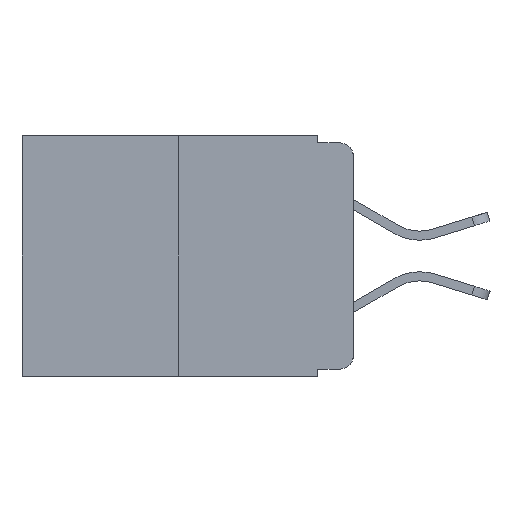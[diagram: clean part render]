
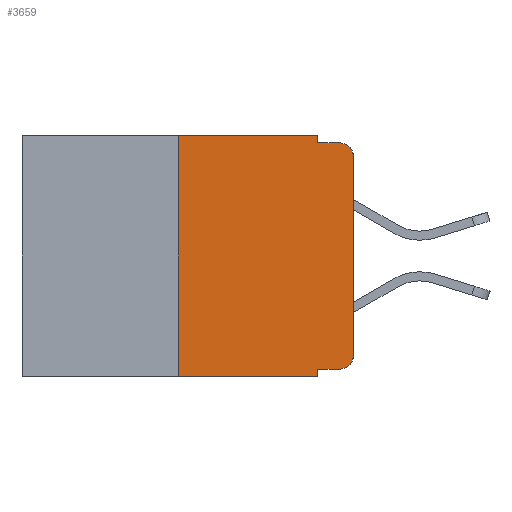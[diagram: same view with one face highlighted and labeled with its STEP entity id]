
A CAD part, left-side view. The second image highlights one B-rep face of the part: STEP entity #3659.
In plain terms, the highlighted planar face has unit normal (-1, 0, 0).
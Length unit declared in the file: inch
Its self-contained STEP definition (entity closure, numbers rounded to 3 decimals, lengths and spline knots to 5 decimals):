
#132 = VERTEX_POINT ( 'NONE', #7792 ) ;
#161 = CARTESIAN_POINT ( 'NONE',  ( 0., 0.473, 0. ) ) ;
#556 = CARTESIAN_POINT ( 'NONE',  ( 0., 0.02, -0.03 ) ) ;
#569 = FACE_OUTER_BOUND ( 'NONE', #10077, .T. ) ;
#776 = VECTOR ( 'NONE', #2933, 39.37008 ) ;
#932 = AXIS2_PLACEMENT_3D ( 'NONE', #6348, #8882, #5397 ) ;
#1039 = LINE ( 'NONE', #8646, #12114 ) ;
#1228 = VERTEX_POINT ( 'NONE', #4421 ) ;
#1411 = VERTEX_POINT ( 'NONE', #13259 ) ;
#1465 = VERTEX_POINT ( 'NONE', #2578 ) ;
#1787 = CIRCLE ( 'NONE', #10687, 0.02 ) ;
#1833 = CARTESIAN_POINT ( 'NONE',  ( 0., 0.25, -0.343 ) ) ;
#1888 = DIRECTION ( 'NONE',  ( -1., 0., 0. ) ) ;
#2293 = LINE ( 'NONE', #7137, #13174 ) ;
#2578 = CARTESIAN_POINT ( 'NONE',  ( 0., 0.051, -0.333 ) ) ;
#2852 = PLANE ( 'NONE',  #932 ) ;
#2933 = DIRECTION ( 'NONE',  ( 0., -1., 0. ) ) ;
#2960 = VERTEX_POINT ( 'NONE', #14194 ) ;
#3230 = DIRECTION ( 'NONE',  ( 0., -1., 0. ) ) ;
#3345 = DIRECTION ( 'NONE',  ( 0., -1., 0. ) ) ;
#3346 = ORIENTED_EDGE ( 'NONE', *, *, #15457, .T. ) ;
#3429 = VERTEX_POINT ( 'NONE', #15495 ) ;
#3498 = EDGE_CURVE ( 'NONE', #1465, #132, #1039, .T. ) ;
#3659 = ADVANCED_FACE ( 'NONE', ( #569 ), #2852, .F. ) ;
#3873 = DIRECTION ( 'NONE',  ( 0., -1., 0. ) ) ;
#4078 = VERTEX_POINT ( 'NONE', #8947 ) ;
#4104 = EDGE_CURVE ( 'NONE', #2960, #1411, #14764, .T. ) ;
#4209 = ORIENTED_EDGE ( 'NONE', *, *, #6328, .F. ) ;
#4421 = CARTESIAN_POINT ( 'NONE',  ( 0., 0.051, 0. ) ) ;
#4448 = CARTESIAN_POINT ( 'NONE',  ( 0., 0.051, -0.01 ) ) ;
#4771 = DIRECTION ( 'NONE',  ( 0., 0., -1. ) ) ;
#4824 = ORIENTED_EDGE ( 'NONE', *, *, #7489, .F. ) ;
#5397 = DIRECTION ( 'NONE',  ( 0., 0., -1. ) ) ;
#5861 = CARTESIAN_POINT ( 'NONE',  ( 0., 0.25, 0. ) ) ;
#6328 = EDGE_CURVE ( 'NONE', #11971, #1228, #12400, .T. ) ;
#6348 = CARTESIAN_POINT ( 'NONE',  ( 0., 0.473, 0. ) ) ;
#6651 = CARTESIAN_POINT ( 'NONE',  ( 0., 0.02, -0.313 ) ) ;
#6722 = EDGE_CURVE ( 'NONE', #1465, #3429, #2293, .T. ) ;
#6922 = LINE ( 'NONE', #7237, #15453 ) ;
#7137 = CARTESIAN_POINT ( 'NONE',  ( 0., 0.051, -0.333 ) ) ;
#7237 = CARTESIAN_POINT ( 'NONE',  ( 0., 0.051, -0.01 ) ) ;
#7474 = LINE ( 'NONE', #9709, #8075 ) ;
#7489 = EDGE_CURVE ( 'NONE', #11614, #4078, #6922, .T. ) ;
#7792 = CARTESIAN_POINT ( 'NONE',  ( 0., 0.051, -0.343 ) ) ;
#8075 = VECTOR ( 'NONE', #4771, 39.37008 ) ;
#8183 = DIRECTION ( 'NONE',  ( 0., 0., 1. ) ) ;
#8496 = DIRECTION ( 'NONE',  ( 0., 0., -1. ) ) ;
#8646 = CARTESIAN_POINT ( 'NONE',  ( 0., 0.051, 0. ) ) ;
#8857 = CARTESIAN_POINT ( 'NONE',  ( 0., 0., 0. ) ) ;
#8882 = DIRECTION ( 'NONE',  ( 1., 0., 0. ) ) ;
#8947 = CARTESIAN_POINT ( 'NONE',  ( 0., 0.02, -0.01 ) ) ;
#9709 = CARTESIAN_POINT ( 'NONE',  ( 0., 0.051, 0. ) ) ;
#10041 = ORIENTED_EDGE ( 'NONE', *, *, #15608, .T. ) ;
#10077 = EDGE_LOOP ( 'NONE', ( #14205, #3346, #4824, #14193, #4209, #14631, #15285, #15186, #13068, #10041 ) ) ;
#10343 = CARTESIAN_POINT ( 'NONE',  ( 0., 0.473, -0.343 ) ) ;
#10425 = LINE ( 'NONE', #10343, #776 ) ;
#10662 = LINE ( 'NONE', #14398, #12459 ) ;
#10687 = AXIS2_PLACEMENT_3D ( 'NONE', #556, #1888, #12798 ) ;
#11300 = VERTEX_POINT ( 'NONE', #1833 ) ;
#11358 = DIRECTION ( 'NONE',  ( 0., 0., 1. ) ) ;
#11540 = DIRECTION ( 'NONE',  ( -1., 0., 0. ) ) ;
#11614 = VERTEX_POINT ( 'NONE', #4448 ) ;
#11726 = AXIS2_PLACEMENT_3D ( 'NONE', #6651, #11540, #15547 ) ;
#11971 = VERTEX_POINT ( 'NONE', #5861 ) ;
#12114 = VECTOR ( 'NONE', #8496, 39.37008 ) ;
#12400 = LINE ( 'NONE', #161, #15159 ) ;
#12459 = VECTOR ( 'NONE', #8183, 39.37008 ) ;
#12690 = EDGE_CURVE ( 'NONE', #1228, #11614, #7474, .T. ) ;
#12798 = DIRECTION ( 'NONE',  ( 0., 0., -1. ) ) ;
#13068 = ORIENTED_EDGE ( 'NONE', *, *, #6722, .T. ) ;
#13174 = VECTOR ( 'NONE', #3230, 39.37008 ) ;
#13246 = CIRCLE ( 'NONE', #11726, 0.02 ) ;
#13259 = CARTESIAN_POINT ( 'NONE',  ( 0., 0., -0.03 ) ) ;
#13664 = EDGE_CURVE ( 'NONE', #11300, #132, #10425, .T. ) ;
#14193 = ORIENTED_EDGE ( 'NONE', *, *, #12690, .F. ) ;
#14194 = CARTESIAN_POINT ( 'NONE',  ( 0., 0., -0.313 ) ) ;
#14205 = ORIENTED_EDGE ( 'NONE', *, *, #4104, .T. ) ;
#14398 = CARTESIAN_POINT ( 'NONE',  ( 0., 0.25, 0. ) ) ;
#14631 = ORIENTED_EDGE ( 'NONE', *, *, #15185, .F. ) ;
#14764 = LINE ( 'NONE', #8857, #14906 ) ;
#14906 = VECTOR ( 'NONE', #11358, 39.37008 ) ;
#15159 = VECTOR ( 'NONE', #3873, 39.37008 ) ;
#15185 = EDGE_CURVE ( 'NONE', #11300, #11971, #10662, .T. ) ;
#15186 = ORIENTED_EDGE ( 'NONE', *, *, #3498, .F. ) ;
#15285 = ORIENTED_EDGE ( 'NONE', *, *, #13664, .T. ) ;
#15453 = VECTOR ( 'NONE', #3345, 39.37008 ) ;
#15457 = EDGE_CURVE ( 'NONE', #1411, #4078, #1787, .T. ) ;
#15495 = CARTESIAN_POINT ( 'NONE',  ( 0., 0.02, -0.333 ) ) ;
#15547 = DIRECTION ( 'NONE',  ( 0., 0., -1. ) ) ;
#15608 = EDGE_CURVE ( 'NONE', #3429, #2960, #13246, .T. ) ;
